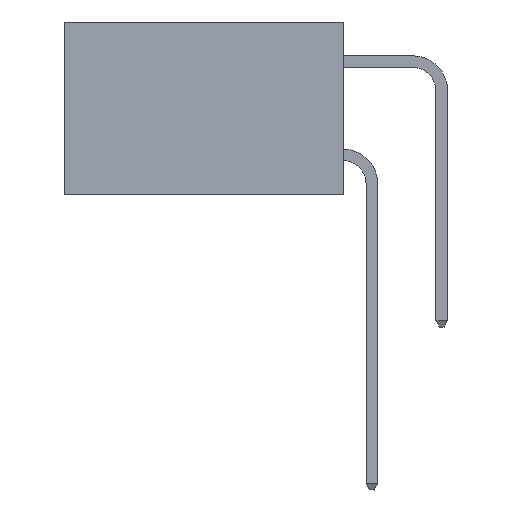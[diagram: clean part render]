
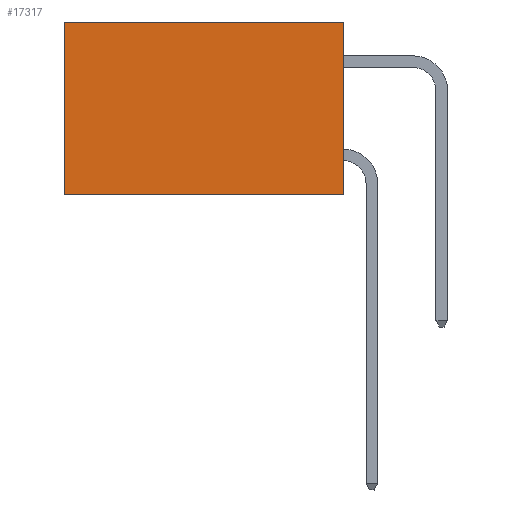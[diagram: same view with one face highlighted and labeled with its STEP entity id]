
A CAD part, left-side view. The second image highlights one B-rep face of the part: STEP entity #17317.
In plain terms, the highlighted planar face has unit normal (-1, 0, 0).
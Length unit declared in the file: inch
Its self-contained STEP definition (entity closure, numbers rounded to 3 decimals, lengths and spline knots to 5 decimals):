
#661 = AXIS2_PLACEMENT_3D ( 'NONE', #15225, #11935, #13643 ) ;
#907 = CARTESIAN_POINT ( 'NONE',  ( 0.2615, 0.6, -0.37 ) ) ;
#2248 = EDGE_CURVE ( 'NONE', #11735, #17685, #22133, .T. ) ;
#2271 = EDGE_CURVE ( 'NONE', #5206, #18027, #17132, .T. ) ;
#2700 = LINE ( 'NONE', #11430, #15244 ) ;
#2968 = CARTESIAN_POINT ( 'NONE',  ( 0.2615, 0.6, -0.37 ) ) ;
#3607 = DIRECTION ( 'NONE',  ( 0., 1., 0. ) ) ;
#4124 = ORIENTED_EDGE ( 'NONE', *, *, #2271, .T. ) ;
#4247 = EDGE_CURVE ( 'NONE', #11735, #5206, #19159, .T. ) ;
#4442 = CARTESIAN_POINT ( 'NONE',  ( 0.2615, 0., -0.37 ) ) ;
#5206 = VERTEX_POINT ( 'NONE', #21157 ) ;
#6723 = DIRECTION ( 'NONE',  ( 0., 0., -1. ) ) ;
#6957 = VECTOR ( 'NONE', #3607, 39.37008 ) ;
#8326 = FACE_OUTER_BOUND ( 'NONE', #9973, .T. ) ;
#9540 = VECTOR ( 'NONE', #6723, 39.37008 ) ;
#9973 = EDGE_LOOP ( 'NONE', ( #4124, #21617, #19737, #17142 ) ) ;
#10803 = EDGE_CURVE ( 'NONE', #17685, #18027, #2700, .T. ) ;
#11430 = CARTESIAN_POINT ( 'NONE',  ( 0.2615, 0., -0.37 ) ) ;
#11727 = VECTOR ( 'NONE', #15094, 39.37008 ) ;
#11735 = VERTEX_POINT ( 'NONE', #19778 ) ;
#11806 = CARTESIAN_POINT ( 'NONE',  ( 0.2615, 0., -0.37 ) ) ;
#11935 = DIRECTION ( 'NONE',  ( 1., 0., 0. ) ) ;
#12276 = PLANE ( 'NONE',  #661 ) ;
#13465 = DIRECTION ( 'NONE',  ( 0., 1., 0. ) ) ;
#13643 = DIRECTION ( 'NONE',  ( 0., 0., -1. ) ) ;
#15094 = DIRECTION ( 'NONE',  ( 0., 0., -1. ) ) ;
#15225 = CARTESIAN_POINT ( 'NONE',  ( 0.2615, 0., -0.37 ) ) ;
#15244 = VECTOR ( 'NONE', #13465, 39.37008 ) ;
#17132 = LINE ( 'NONE', #2968, #9540 ) ;
#17142 = ORIENTED_EDGE ( 'NONE', *, *, #4247, .T. ) ;
#17317 = ADVANCED_FACE ( 'NONE', ( #8326 ), #12276, .F. ) ;
#17685 = VERTEX_POINT ( 'NONE', #4442 ) ;
#18027 = VERTEX_POINT ( 'NONE', #907 ) ;
#19159 = LINE ( 'NONE', #19282, #6957 ) ;
#19282 = CARTESIAN_POINT ( 'NONE',  ( 0.2615, 0., 0. ) ) ;
#19737 = ORIENTED_EDGE ( 'NONE', *, *, #2248, .F. ) ;
#19778 = CARTESIAN_POINT ( 'NONE',  ( 0.2615, 0., 0. ) ) ;
#21157 = CARTESIAN_POINT ( 'NONE',  ( 0.2615, 0.6, 0. ) ) ;
#21617 = ORIENTED_EDGE ( 'NONE', *, *, #10803, .F. ) ;
#22133 = LINE ( 'NONE', #11806, #11727 ) ;
